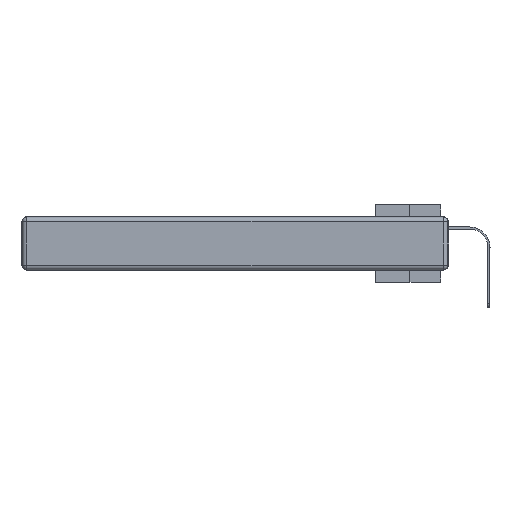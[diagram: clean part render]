
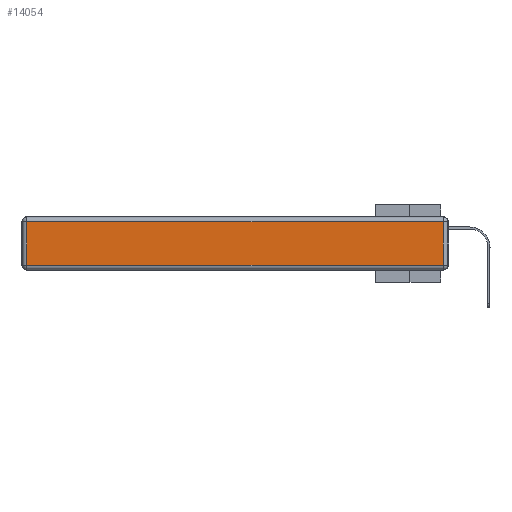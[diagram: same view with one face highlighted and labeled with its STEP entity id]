
A CAD part, left-side view. The second image highlights one B-rep face of the part: STEP entity #14054.
In plain terms, the highlighted planar face has unit normal (-1, 0, 0).
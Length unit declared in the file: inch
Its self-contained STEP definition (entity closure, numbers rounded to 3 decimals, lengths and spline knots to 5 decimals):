
#70 = CARTESIAN_POINT ( 'NONE',  ( 0., 0.03, -0.03 ) ) ;
#2157 = DIRECTION ( 'NONE',  ( -1., 0., 0. ) ) ;
#4573 = DIRECTION ( 'NONE',  ( 0., -1., 0. ) ) ;
#4701 = EDGE_CURVE ( 'NONE', #17232, #38099, #10511, .T. ) ;
#4738 = FACE_OUTER_BOUND ( 'NONE', #30644, .T. ) ;
#5136 = VECTOR ( 'NONE', #17922, 39.37008 ) ;
#6798 = EDGE_CURVE ( 'NONE', #38099, #27766, #6868, .T. ) ;
#6868 = LINE ( 'NONE', #18492, #14600 ) ;
#7888 = CARTESIAN_POINT ( 'NONE',  ( 0., 0., -0.343 ) ) ;
#8432 = CARTESIAN_POINT ( 'NONE',  ( 0., 2.72, -0.313 ) ) ;
#8847 = LINE ( 'NONE', #29481, #5136 ) ;
#10511 = LINE ( 'NONE', #29338, #15904 ) ;
#11850 = VERTEX_POINT ( 'NONE', #16270 ) ;
#14054 = ADVANCED_FACE ( 'NONE', ( #4738 ), #23042, .T. ) ;
#14214 = EDGE_CURVE ( 'NONE', #11850, #17232, #8847, .T. ) ;
#14600 = VECTOR ( 'NONE', #30462, 39.37008 ) ;
#15904 = VECTOR ( 'NONE', #4573, 39.37008 ) ;
#16270 = CARTESIAN_POINT ( 'NONE',  ( 0., 2.72, -0.03 ) ) ;
#17232 = VERTEX_POINT ( 'NONE', #8432 ) ;
#17922 = DIRECTION ( 'NONE',  ( 0., 0., -1. ) ) ;
#18183 = CARTESIAN_POINT ( 'NONE',  ( 0., 0.03, -0.313 ) ) ;
#18343 = AXIS2_PLACEMENT_3D ( 'NONE', #7888, #2157, #34613 ) ;
#18489 = CARTESIAN_POINT ( 'NONE',  ( 0., 2.75, -0.03 ) ) ;
#18492 = CARTESIAN_POINT ( 'NONE',  ( 0., 0.03, -0.343 ) ) ;
#20157 = ORIENTED_EDGE ( 'NONE', *, *, #6798, .T. ) ;
#21630 = LINE ( 'NONE', #18489, #30109 ) ;
#22151 = ORIENTED_EDGE ( 'NONE', *, *, #4701, .T. ) ;
#23042 = PLANE ( 'NONE',  #18343 ) ;
#26052 = ORIENTED_EDGE ( 'NONE', *, *, #14214, .T. ) ;
#27220 = ORIENTED_EDGE ( 'NONE', *, *, #33003, .T. ) ;
#27766 = VERTEX_POINT ( 'NONE', #70 ) ;
#29338 = CARTESIAN_POINT ( 'NONE',  ( 0., 0., -0.313 ) ) ;
#29481 = CARTESIAN_POINT ( 'NONE',  ( 0., 2.72, -0.343 ) ) ;
#30109 = VECTOR ( 'NONE', #33015, 39.37008 ) ;
#30462 = DIRECTION ( 'NONE',  ( 0., 0., 1. ) ) ;
#30644 = EDGE_LOOP ( 'NONE', ( #22151, #20157, #27220, #26052 ) ) ;
#33003 = EDGE_CURVE ( 'NONE', #27766, #11850, #21630, .T. ) ;
#33015 = DIRECTION ( 'NONE',  ( 0., 1., 0. ) ) ;
#34613 = DIRECTION ( 'NONE',  ( 0., 0., 1. ) ) ;
#38099 = VERTEX_POINT ( 'NONE', #18183 ) ;
